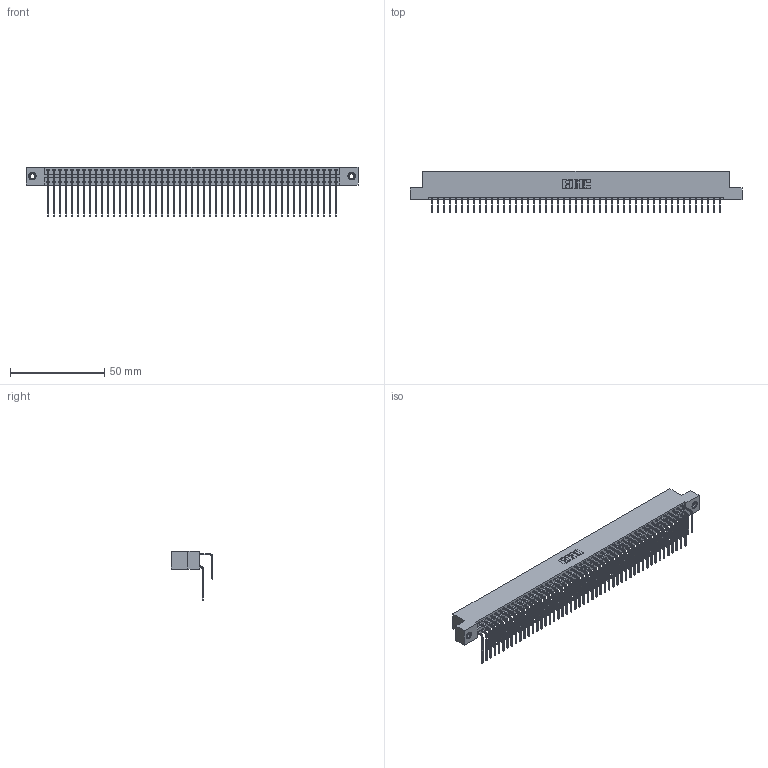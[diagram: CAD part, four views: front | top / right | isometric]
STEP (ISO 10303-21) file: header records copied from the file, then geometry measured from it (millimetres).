
FILE_DESCRIPTION (( 'STEP AP203' ), '1' );
FILE_NAME ('346-098-558-207.STEP', '2022-05-26T19:04:48', ( '' ), ( '' ), 'SwSTEP 2.0', 'SolidWorks 2020', '' );
FILE_SCHEMA (( 'CONFIG_CONTROL_DESIGN' ));
Length unit declared in the file: inch
Products named in the file (5): 345-250-001_345-250-005-103; 345-292-001_558 Tail - 2; 345-292-001_558 559 Tail - 1; 346 Part_Flush Mounting Lugs - 0.156 Dia-TI; 346-098-558-207
Assembly tree (101 placements, depth 2):
  346-098-558-207
    346 Part_Flush Mounting Lugs - 0.156 Dia-TI
    345-292-001_558 559 Tail - 1  x49
    345-292-001_558 Tail - 2  x49
    345-250-001_345-250-005-103  x2
Bounding box: 176.15 x 22.16 x 26.16 mm (x, y, z)
Volume: 17782.9 mm3; surface area: 27299.7 mm2
Topology: 101 solids, 101 shells, 5474 faces, 16243 edges, 10690 vertices
Faces by surface type: plane 3734, cylinder 1724, cone 12, torus 4
Entity records: 34006 total; most frequent: CARTESIAN_POINT 5630, ORIENTED_EDGE 5506, DIRECTION 5011, EDGE_CURVE 2753, VECTOR 2365, LINE 2365, VERTEX_POINT 1828, AXIS2_PLACEMENT_3D 1323
